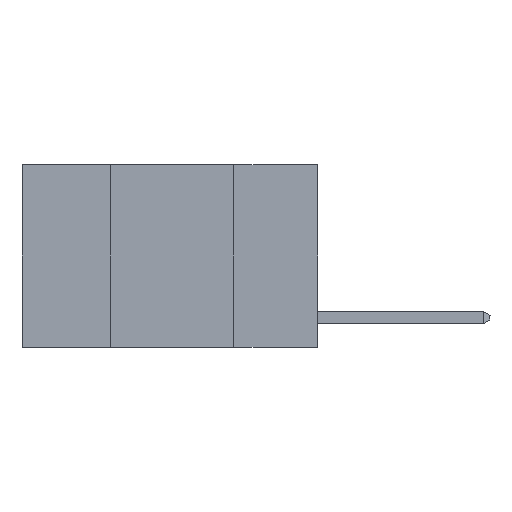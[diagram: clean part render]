
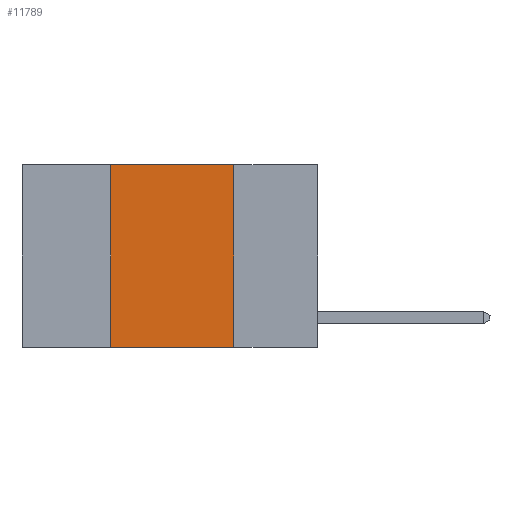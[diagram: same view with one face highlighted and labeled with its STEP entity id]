
A CAD part, left-side view. The second image highlights one B-rep face of the part: STEP entity #11789.
In plain terms, the highlighted planar face has unit normal (-1, 0, 0).
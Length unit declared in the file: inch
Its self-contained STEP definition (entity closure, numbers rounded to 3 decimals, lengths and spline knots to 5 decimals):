
#163 = CARTESIAN_POINT ( 'NONE',  ( 0., 0.17, 0. ) ) ;
#511 = CARTESIAN_POINT ( 'NONE',  ( 0., 0.6, -0.37 ) ) ;
#598 = VECTOR ( 'NONE', #3355, 39.37008 ) ;
#823 = LINE ( 'NONE', #21024, #1479 ) ;
#1479 = VECTOR ( 'NONE', #7408, 39.37008 ) ;
#2671 = ORIENTED_EDGE ( 'NONE', *, *, #19976, .T. ) ;
#2705 = VERTEX_POINT ( 'NONE', #10346 ) ;
#2959 = ORIENTED_EDGE ( 'NONE', *, *, #5013, .F. ) ;
#3355 = DIRECTION ( 'NONE',  ( 0., 0., -1. ) ) ;
#5013 = EDGE_CURVE ( 'NONE', #2705, #12853, #27441, .T. ) ;
#5133 = EDGE_CURVE ( 'NONE', #27527, #15934, #23693, .T. ) ;
#5744 = LINE ( 'NONE', #511, #5951 ) ;
#5951 = VECTOR ( 'NONE', #14293, 39.37008 ) ;
#6686 = AXIS2_PLACEMENT_3D ( 'NONE', #28113, #7629, #18887 ) ;
#7408 = DIRECTION ( 'NONE',  ( 0., -1., 0. ) ) ;
#7629 = DIRECTION ( 'NONE',  ( 1., 0., 0. ) ) ;
#9645 = DIRECTION ( 'NONE',  ( 0., 0., 1. ) ) ;
#9807 = CARTESIAN_POINT ( 'NONE',  ( 0., 0.42, 0. ) ) ;
#10155 = VECTOR ( 'NONE', #9645, 39.37008 ) ;
#10346 = CARTESIAN_POINT ( 'NONE',  ( 0., 0.42, -0.37 ) ) ;
#11789 = ADVANCED_FACE ( 'NONE', ( #23773 ), #21400, .F. ) ;
#12754 = EDGE_CURVE ( 'NONE', #12853, #27527, #823, .T. ) ;
#12853 = VERTEX_POINT ( 'NONE', #9807 ) ;
#14293 = DIRECTION ( 'NONE',  ( 0., -1., 0. ) ) ;
#15934 = VERTEX_POINT ( 'NONE', #24703 ) ;
#18887 = DIRECTION ( 'NONE',  ( 0., 0., -1. ) ) ;
#19101 = EDGE_LOOP ( 'NONE', ( #29042, #22058, #2959, #2671 ) ) ;
#19392 = CARTESIAN_POINT ( 'NONE',  ( 0., 0.17, 0. ) ) ;
#19976 = EDGE_CURVE ( 'NONE', #2705, #15934, #5744, .T. ) ;
#20723 = CARTESIAN_POINT ( 'NONE',  ( 0., 0.42, 0. ) ) ;
#21024 = CARTESIAN_POINT ( 'NONE',  ( 0., 0.6, 0. ) ) ;
#21400 = PLANE ( 'NONE',  #6686 ) ;
#22058 = ORIENTED_EDGE ( 'NONE', *, *, #12754, .F. ) ;
#23693 = LINE ( 'NONE', #19392, #598 ) ;
#23773 = FACE_OUTER_BOUND ( 'NONE', #19101, .T. ) ;
#24703 = CARTESIAN_POINT ( 'NONE',  ( 0., 0.17, -0.37 ) ) ;
#27441 = LINE ( 'NONE', #20723, #10155 ) ;
#27527 = VERTEX_POINT ( 'NONE', #163 ) ;
#28113 = CARTESIAN_POINT ( 'NONE',  ( 0., 0.6, 0. ) ) ;
#29042 = ORIENTED_EDGE ( 'NONE', *, *, #5133, .F. ) ;
